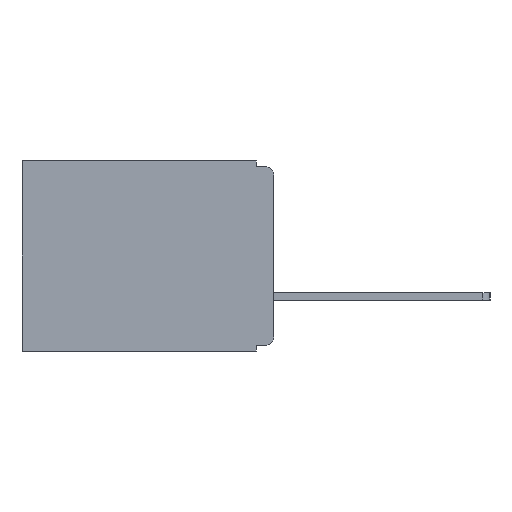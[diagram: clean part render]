
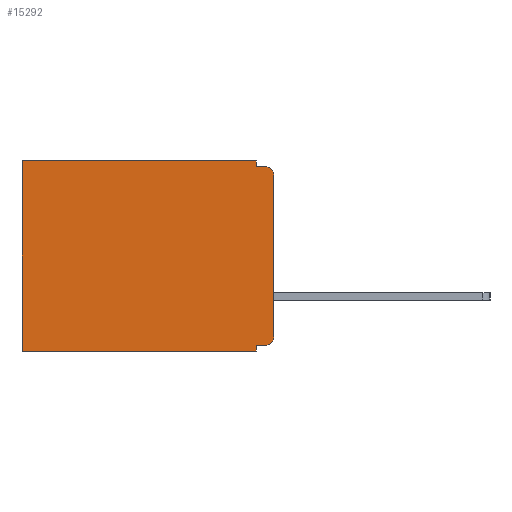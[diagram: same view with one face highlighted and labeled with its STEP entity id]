
A CAD part, left-side view. The second image highlights one B-rep face of the part: STEP entity #15292.
In plain terms, the highlighted planar face has unit normal (-1, 0, 0).
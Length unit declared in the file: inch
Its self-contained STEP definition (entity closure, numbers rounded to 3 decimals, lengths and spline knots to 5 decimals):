
#284 = VERTEX_POINT ( 'NONE', #16709 ) ;
#412 = ORIENTED_EDGE ( 'NONE', *, *, #5062, .F. ) ;
#420 = CARTESIAN_POINT ( 'NONE',  ( 0.3, 0.437, -0.33 ) ) ;
#541 = EDGE_CURVE ( 'NONE', #13186, #284, #7107, .T. ) ;
#544 = VECTOR ( 'NONE', #7188, 39.37008 ) ;
#574 = VERTEX_POINT ( 'NONE', #5919 ) ;
#965 = EDGE_CURVE ( 'NONE', #13680, #284, #19247, .T. ) ;
#1489 = VECTOR ( 'NONE', #18341, 39.37008 ) ;
#1507 = ORIENTED_EDGE ( 'NONE', *, *, #10639, .T. ) ;
#1561 = CARTESIAN_POINT ( 'NONE',  ( 0.3, 0.015, -0.01 ) ) ;
#1768 = CARTESIAN_POINT ( 'NONE',  ( 0.3, 0., -0.33 ) ) ;
#2117 = LINE ( 'NONE', #17073, #18037 ) ;
#2147 = DIRECTION ( 'NONE',  ( -1., 0., 0. ) ) ;
#2204 = LINE ( 'NONE', #6013, #10518 ) ;
#2520 = DIRECTION ( 'NONE',  ( 0., 1., 0. ) ) ;
#2588 = EDGE_CURVE ( 'NONE', #13327, #574, #2117, .T. ) ;
#2917 = EDGE_CURVE ( 'NONE', #13186, #8700, #8235, .T. ) ;
#3520 = VECTOR ( 'NONE', #14989, 39.37008 ) ;
#3613 = DIRECTION ( 'NONE',  ( 0., 0., -1. ) ) ;
#4205 = VERTEX_POINT ( 'NONE', #420 ) ;
#4321 = CARTESIAN_POINT ( 'NONE',  ( 0.3, 0.015, -0.305 ) ) ;
#4340 = VECTOR ( 'NONE', #13320, 39.37008 ) ;
#4443 = ORIENTED_EDGE ( 'NONE', *, *, #15287, .F. ) ;
#4460 = ORIENTED_EDGE ( 'NONE', *, *, #8039, .F. ) ;
#4817 = AXIS2_PLACEMENT_3D ( 'NONE', #4321, #2147, #16837 ) ;
#4827 = ORIENTED_EDGE ( 'NONE', *, *, #13176, .T. ) ;
#5062 = EDGE_CURVE ( 'NONE', #8192, #4205, #9463, .T. ) ;
#5558 = ORIENTED_EDGE ( 'NONE', *, *, #965, .F. ) ;
#5648 = CARTESIAN_POINT ( 'NONE',  ( 0.3, 0.437, -0.33 ) ) ;
#5698 = LINE ( 'NONE', #7556, #1489 ) ;
#5919 = CARTESIAN_POINT ( 'NONE',  ( 0.3, 0.437, 0. ) ) ;
#6013 = CARTESIAN_POINT ( 'NONE',  ( 0.3, 0.031, 0. ) ) ;
#6064 = ORIENTED_EDGE ( 'NONE', *, *, #2917, .F. ) ;
#6410 = CARTESIAN_POINT ( 'NONE',  ( 0.3, 0.015, -0.025 ) ) ;
#7107 = CIRCLE ( 'NONE', #4817, 0.015 ) ;
#7188 = DIRECTION ( 'NONE',  ( 0., 0., -1. ) ) ;
#7519 = PLANE ( 'NONE',  #10346 ) ;
#7556 = CARTESIAN_POINT ( 'NONE',  ( 0.3, 0., -0.01 ) ) ;
#7558 = DIRECTION ( 'NONE',  ( 0., 1., 0. ) ) ;
#7835 = CARTESIAN_POINT ( 'NONE',  ( 0.3, 0., -0.32 ) ) ;
#7952 = DIRECTION ( 'NONE',  ( 0., 0., -1. ) ) ;
#8039 = EDGE_CURVE ( 'NONE', #11883, #13702, #5698, .T. ) ;
#8192 = VERTEX_POINT ( 'NONE', #14162 ) ;
#8235 = LINE ( 'NONE', #7835, #19407 ) ;
#8700 = VERTEX_POINT ( 'NONE', #18323 ) ;
#9110 = DIRECTION ( 'NONE',  ( 0., 0., -1. ) ) ;
#9365 = LINE ( 'NONE', #5648, #544 ) ;
#9370 = CARTESIAN_POINT ( 'NONE',  ( 0.3, 0., -0.025 ) ) ;
#9463 = LINE ( 'NONE', #13789, #4340 ) ;
#9933 = EDGE_LOOP ( 'NONE', ( #5558, #1507, #4460, #4443, #11643, #4827, #412, #16456, #6064, #12791 ) ) ;
#10034 = FACE_OUTER_BOUND ( 'NONE', #9933, .T. ) ;
#10346 = AXIS2_PLACEMENT_3D ( 'NONE', #13668, #18235, #9110 ) ;
#10518 = VECTOR ( 'NONE', #15182, 39.37008 ) ;
#10639 = EDGE_CURVE ( 'NONE', #13680, #13702, #15463, .T. ) ;
#11643 = ORIENTED_EDGE ( 'NONE', *, *, #2588, .T. ) ;
#11883 = VERTEX_POINT ( 'NONE', #14581 ) ;
#12640 = EDGE_CURVE ( 'NONE', #8700, #8192, #14418, .T. ) ;
#12739 = AXIS2_PLACEMENT_3D ( 'NONE', #6410, #17134, #7952 ) ;
#12791 = ORIENTED_EDGE ( 'NONE', *, *, #541, .T. ) ;
#13176 = EDGE_CURVE ( 'NONE', #574, #4205, #9365, .T. ) ;
#13186 = VERTEX_POINT ( 'NONE', #19384 ) ;
#13320 = DIRECTION ( 'NONE',  ( 0., 1., 0. ) ) ;
#13327 = VERTEX_POINT ( 'NONE', #15036 ) ;
#13668 = CARTESIAN_POINT ( 'NONE',  ( 0.3, 0., -0.33 ) ) ;
#13680 = VERTEX_POINT ( 'NONE', #9370 ) ;
#13702 = VERTEX_POINT ( 'NONE', #1561 ) ;
#13789 = CARTESIAN_POINT ( 'NONE',  ( 0.3, 0., -0.33 ) ) ;
#14162 = CARTESIAN_POINT ( 'NONE',  ( 0.3, 0.031, -0.33 ) ) ;
#14418 = LINE ( 'NONE', #19529, #3520 ) ;
#14581 = CARTESIAN_POINT ( 'NONE',  ( 0.3, 0.031, -0.01 ) ) ;
#14786 = VECTOR ( 'NONE', #3613, 39.37008 ) ;
#14989 = DIRECTION ( 'NONE',  ( 0., 0., -1. ) ) ;
#15036 = CARTESIAN_POINT ( 'NONE',  ( 0.3, 0.031, 0. ) ) ;
#15182 = DIRECTION ( 'NONE',  ( 0., 0., -1. ) ) ;
#15287 = EDGE_CURVE ( 'NONE', #13327, #11883, #2204, .T. ) ;
#15292 = ADVANCED_FACE ( 'NONE', ( #10034 ), #7519, .F. ) ;
#15463 = CIRCLE ( 'NONE', #12739, 0.015 ) ;
#16456 = ORIENTED_EDGE ( 'NONE', *, *, #12640, .F. ) ;
#16709 = CARTESIAN_POINT ( 'NONE',  ( 0.3, 0., -0.305 ) ) ;
#16837 = DIRECTION ( 'NONE',  ( 0., 0., -1. ) ) ;
#17073 = CARTESIAN_POINT ( 'NONE',  ( 0.3, 0., 0. ) ) ;
#17134 = DIRECTION ( 'NONE',  ( -1., 0., 0. ) ) ;
#18037 = VECTOR ( 'NONE', #2520, 39.37008 ) ;
#18235 = DIRECTION ( 'NONE',  ( 1., 0., 0. ) ) ;
#18323 = CARTESIAN_POINT ( 'NONE',  ( 0.3, 0.031, -0.32 ) ) ;
#18341 = DIRECTION ( 'NONE',  ( 0., -1., 0. ) ) ;
#19247 = LINE ( 'NONE', #1768, #14786 ) ;
#19384 = CARTESIAN_POINT ( 'NONE',  ( 0.3, 0.015, -0.32 ) ) ;
#19407 = VECTOR ( 'NONE', #7558, 39.37008 ) ;
#19529 = CARTESIAN_POINT ( 'NONE',  ( 0.3, 0.031, -0.33 ) ) ;
